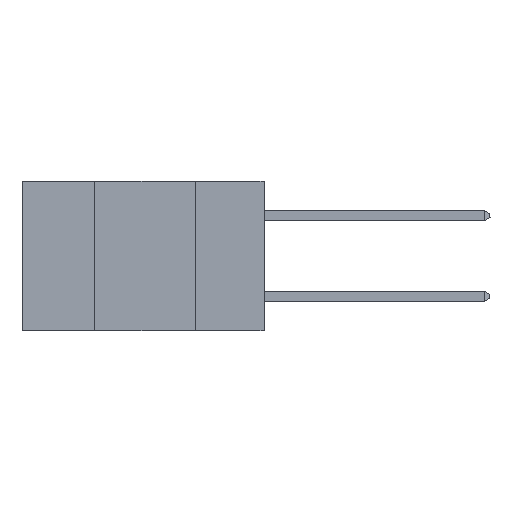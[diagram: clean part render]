
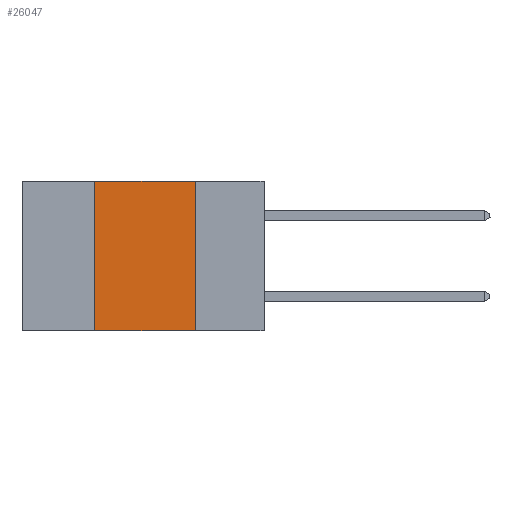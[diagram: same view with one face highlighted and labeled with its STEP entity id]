
A CAD part, left-side view. The second image highlights one B-rep face of the part: STEP entity #26047.
In plain terms, the highlighted planar face has unit normal (-1, 0, 0).
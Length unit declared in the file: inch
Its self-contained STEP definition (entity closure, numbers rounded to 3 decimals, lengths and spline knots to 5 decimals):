
#540 = VECTOR ( 'NONE', #23892, 39.37008 ) ;
#596 = ORIENTED_EDGE ( 'NONE', *, *, #9472, .F. ) ;
#1103 = VERTEX_POINT ( 'NONE', #12160 ) ;
#1402 = LINE ( 'NONE', #28365, #27110 ) ;
#1871 = VERTEX_POINT ( 'NONE', #18931 ) ;
#2202 = EDGE_CURVE ( 'NONE', #1103, #11434, #9956, .T. ) ;
#3948 = DIRECTION ( 'NONE',  ( 0., 0., 1. ) ) ;
#4555 = EDGE_CURVE ( 'NONE', #1871, #11434, #1402, .T. ) ;
#6512 = FACE_OUTER_BOUND ( 'NONE', #24476, .T. ) ;
#6575 = LINE ( 'NONE', #8074, #16951 ) ;
#6642 = CARTESIAN_POINT ( 'NONE',  ( 0., 0.17, 0. ) ) ;
#7499 = LINE ( 'NONE', #23793, #540 ) ;
#8074 = CARTESIAN_POINT ( 'NONE',  ( 0., 0.42, 0. ) ) ;
#8128 = DIRECTION ( 'NONE',  ( 0., 0., -1. ) ) ;
#9472 = EDGE_CURVE ( 'NONE', #15939, #1103, #7499, .T. ) ;
#9956 = LINE ( 'NONE', #6642, #18256 ) ;
#10117 = ORIENTED_EDGE ( 'NONE', *, *, #2202, .F. ) ;
#11434 = VERTEX_POINT ( 'NONE', #15134 ) ;
#12160 = CARTESIAN_POINT ( 'NONE',  ( 0., 0.17, 0. ) ) ;
#13090 = EDGE_CURVE ( 'NONE', #1871, #15939, #6575, .T. ) ;
#14019 = CARTESIAN_POINT ( 'NONE',  ( 0., 0.42, 0. ) ) ;
#15134 = CARTESIAN_POINT ( 'NONE',  ( 0., 0.17, -0.37 ) ) ;
#15939 = VERTEX_POINT ( 'NONE', #14019 ) ;
#16941 = CARTESIAN_POINT ( 'NONE',  ( 0., 0.6, 0. ) ) ;
#16951 = VECTOR ( 'NONE', #3948, 39.37008 ) ;
#17391 = DIRECTION ( 'NONE',  ( 0., 0., -1. ) ) ;
#17432 = DIRECTION ( 'NONE',  ( 0., -1., 0. ) ) ;
#18256 = VECTOR ( 'NONE', #17391, 39.37008 ) ;
#18931 = CARTESIAN_POINT ( 'NONE',  ( 0., 0.42, -0.37 ) ) ;
#19351 = ORIENTED_EDGE ( 'NONE', *, *, #13090, .F. ) ;
#21195 = AXIS2_PLACEMENT_3D ( 'NONE', #16941, #21440, #8128 ) ;
#21440 = DIRECTION ( 'NONE',  ( 1., 0., 0. ) ) ;
#23005 = ORIENTED_EDGE ( 'NONE', *, *, #4555, .T. ) ;
#23793 = CARTESIAN_POINT ( 'NONE',  ( 0., 0.6, 0. ) ) ;
#23892 = DIRECTION ( 'NONE',  ( 0., -1., 0. ) ) ;
#24476 = EDGE_LOOP ( 'NONE', ( #10117, #596, #19351, #23005 ) ) ;
#26047 = ADVANCED_FACE ( 'NONE', ( #6512 ), #27504, .F. ) ;
#27110 = VECTOR ( 'NONE', #17432, 39.37008 ) ;
#27504 = PLANE ( 'NONE',  #21195 ) ;
#28365 = CARTESIAN_POINT ( 'NONE',  ( 0., 0.6, -0.37 ) ) ;
